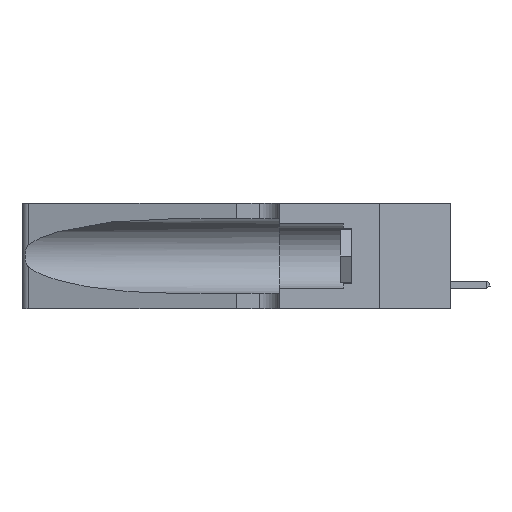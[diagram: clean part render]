
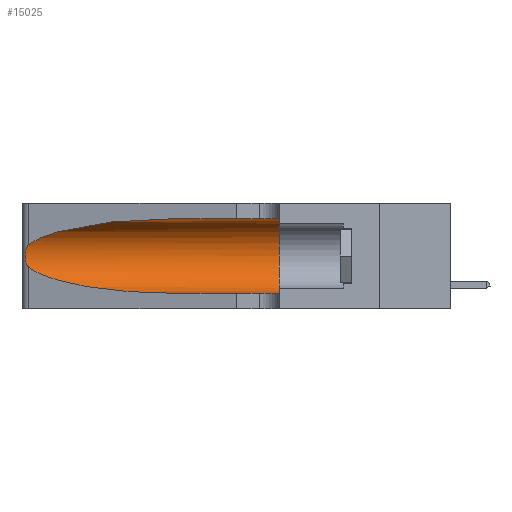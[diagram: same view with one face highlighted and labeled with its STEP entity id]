
A CAD part, left-side view. The second image highlights one B-rep face of the part: STEP entity #15025.
In plain terms, the highlighted cylindrical face has radius 3.308 mm (diameter 6.617 mm), a partial arc.
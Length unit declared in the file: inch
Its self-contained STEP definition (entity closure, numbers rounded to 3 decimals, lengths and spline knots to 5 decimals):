
#577 = CARTESIAN_POINT ( 'NONE',  ( 0.1305, 1.61858, 0.05475 ) ) ;
#926 = CARTESIAN_POINT ( 'NONE',  ( 0.25487, 1.22718, 0.22369 ) ) ;
#1427 = CARTESIAN_POINT ( 'NONE',  ( 0.2373, 1.15595, 0.08982 ) ) ;
#1828 = CARTESIAN_POINT ( 'NONE',  ( 0.25789, 1.23486, 0.15765 ) ) ;
#1886 = CARTESIAN_POINT ( 'NONE',  ( 0.1305, 1.61858, 0.31525 ) ) ;
#2007 = CARTESIAN_POINT ( 'NONE',  ( 0.1305, 0.72297, 0.31525 ) ) ;
#2019 = AXIS2_PLACEMENT_3D ( 'NONE', #18023, #8363, #10877 ) ;
#2122 = EDGE_CURVE ( 'NONE', #17724, #21665, #11173, .T. ) ;
#3225 = CARTESIAN_POINT ( 'NONE',  ( 0.1305, 1.61858, 0.185 ) ) ;
#3258 = EDGE_LOOP ( 'NONE', ( #9719, #6679, #14678, #19673, #24991, #16058 ) ) ;
#5474 = LINE ( 'NONE', #577, #17041 ) ;
#5786 = CARTESIAN_POINT ( 'NONE',  ( 0.25854, 1.2359, 0.20912 ) ) ;
#6450 = AXIS2_PLACEMENT_3D ( 'NONE', #3225, #24688, #18754 ) ;
#6679 = ORIENTED_EDGE ( 'NONE', *, *, #7517, .T. ) ;
#6964 = CARTESIAN_POINT ( 'NONE',  ( 0.1305, 0.35, 0.31525 ) ) ;
#7098 = CARTESIAN_POINT ( 'NONE',  ( 0.18966, 0.96281, 0.05475 ) ) ;
#7517 = EDGE_CURVE ( 'NONE', #14878, #10443, #12636, .T. ) ;
#7521 = CARTESIAN_POINT ( 'NONE',  ( 0.26017, 1.23833, 0.17102 ) ) ;
#7682 = CARTESIAN_POINT ( 'NONE',  ( 0.25856, 1.23593, 0.16098 ) ) ;
#7783 = CARTESIAN_POINT ( 'NONE',  ( 0.18966, 0.96281, 0.31525 ) ) ;
#8119 = CARTESIAN_POINT ( 'NONE',  ( 0.1305, 0.72297, 0.31525 ) ) ;
#8363 = DIRECTION ( 'NONE',  ( 0., 1., 0. ) ) ;
#8421 = FACE_OUTER_BOUND ( 'NONE', #3258, .T. ) ;
#9545 = DIRECTION ( 'NONE',  ( 0., -1., 0. ) ) ;
#9719 = ORIENTED_EDGE ( 'NONE', *, *, #24271, .T. ) ;
#9806 = CARTESIAN_POINT ( 'NONE',  ( 0.25487, 1.22718, 0.14631 ) ) ;
#10043 = EDGE_CURVE ( 'NONE', #21665, #16851, #21026, .T. ) ;
#10149 = EDGE_CURVE ( 'NONE', #14196, #16851, #5474, .T. ) ;
#10443 = VERTEX_POINT ( 'NONE', #12138 ) ;
#10877 = DIRECTION ( 'NONE',  ( 0., 0., 1. ) ) ;
#11173 = LINE ( 'NONE', #1886, #15123 ) ;
#11995 = EDGE_CURVE ( 'NONE', #10443, #14196, #16378, .T. ) ;
#12138 = CARTESIAN_POINT ( 'NONE',  ( 0.25487, 1.22718, 0.14631 ) ) ;
#12348 = CYLINDRICAL_SURFACE ( 'NONE', #6450, 0.13025 ) ;
#12636 = B_SPLINE_CURVE_WITH_KNOTS ( 'NONE', 3,
 ( #17522, #23247, #19146, #19464, #5786, #17267, #23062, #23220, #7521, #7682, #1828, #21189, #21274, #9806 ),
 .UNSPECIFIED., .F., .F.,
 ( 4, 2, 2, 2, 2, 2, 4 ),
 ( 0., 0.00027, 0.00053, 0.00107, 0.0016, 0.00187, 0.00214 ),
 .UNSPECIFIED. ) ;
#14196 = VERTEX_POINT ( 'NONE', #19982 ) ;
#14678 = ORIENTED_EDGE ( 'NONE', *, *, #11995, .T. ) ;
#14878 = VERTEX_POINT ( 'NONE', #926 ) ;
#15025 = ADVANCED_FACE ( 'NONE', ( #8421 ), #12348, .F. ) ;
#15097 = DIRECTION ( 'NONE',  ( 0., -1., 0. ) ) ;
#15123 = VECTOR ( 'NONE', #9545, 39.37008 ) ;
#15824 = CARTESIAN_POINT ( 'NONE',  ( 0.2373, 1.15595, 0.28018 ) ) ;
#16058 = ORIENTED_EDGE ( 'NONE', *, *, #2122, .F. ) ;
#16378 =( BOUNDED_CURVE ( )  B_SPLINE_CURVE ( 3, ( #20607, #1427, #7098, #20696 ),
 .UNSPECIFIED., .F., .F. ) 
 B_SPLINE_CURVE_WITH_KNOTS ( ( 4, 4 ),
 ( 3.44316, 4.71239 ),
 .UNSPECIFIED. ) 
 CURVE ( )  GEOMETRIC_REPRESENTATION_ITEM ( )  RATIONAL_B_SPLINE_CURVE ( ( 1., 0.87, 0.87, 1. ) ) 
 REPRESENTATION_ITEM ( '' )  );
#16851 = VERTEX_POINT ( 'NONE', #18843 ) ;
#17041 = VECTOR ( 'NONE', #15097, 39.37008 ) ;
#17267 = CARTESIAN_POINT ( 'NONE',  ( 0.26018, 1.23835, 0.19895 ) ) ;
#17522 = CARTESIAN_POINT ( 'NONE',  ( 0.25487, 1.22718, 0.22369 ) ) ;
#17724 = VERTEX_POINT ( 'NONE', #8119 ) ;
#18023 = CARTESIAN_POINT ( 'NONE',  ( 0.1305, 0.35, 0.185 ) ) ;
#18705 =( BOUNDED_CURVE ( )  B_SPLINE_CURVE ( 3, ( #2007, #7783, #15824, #19469 ),
 .UNSPECIFIED., .F., .F. ) 
 B_SPLINE_CURVE_WITH_KNOTS ( ( 4, 4 ),
 ( 1.5708, 2.84003 ),
 .UNSPECIFIED. ) 
 CURVE ( )  GEOMETRIC_REPRESENTATION_ITEM ( )  RATIONAL_B_SPLINE_CURVE ( ( 1., 0.87, 0.87, 1. ) ) 
 REPRESENTATION_ITEM ( '' )  );
#18754 = DIRECTION ( 'NONE',  ( 0., 0., -1. ) ) ;
#18843 = CARTESIAN_POINT ( 'NONE',  ( 0.1305, 0.35, 0.05475 ) ) ;
#19146 = CARTESIAN_POINT ( 'NONE',  ( 0.25639, 1.23184, 0.21858 ) ) ;
#19464 = CARTESIAN_POINT ( 'NONE',  ( 0.25787, 1.23484, 0.2124 ) ) ;
#19469 = CARTESIAN_POINT ( 'NONE',  ( 0.25487, 1.22718, 0.22369 ) ) ;
#19673 = ORIENTED_EDGE ( 'NONE', *, *, #10149, .T. ) ;
#19982 = CARTESIAN_POINT ( 'NONE',  ( 0.1305, 0.72297, 0.05475 ) ) ;
#20607 = CARTESIAN_POINT ( 'NONE',  ( 0.25487, 1.22718, 0.14631 ) ) ;
#20696 = CARTESIAN_POINT ( 'NONE',  ( 0.1305, 0.72297, 0.05475 ) ) ;
#21026 = CIRCLE ( 'NONE', #2019, 0.13025 ) ;
#21189 = CARTESIAN_POINT ( 'NONE',  ( 0.25639, 1.23186, 0.15144 ) ) ;
#21274 = CARTESIAN_POINT ( 'NONE',  ( 0.25555, 1.22993, 0.14849 ) ) ;
#21665 = VERTEX_POINT ( 'NONE', #6964 ) ;
#23062 = CARTESIAN_POINT ( 'NONE',  ( 0.26075, 1.23896, 0.19203 ) ) ;
#23220 = CARTESIAN_POINT ( 'NONE',  ( 0.26075, 1.23896, 0.178 ) ) ;
#23247 = CARTESIAN_POINT ( 'NONE',  ( 0.25555, 1.22994, 0.2215 ) ) ;
#24271 = EDGE_CURVE ( 'NONE', #17724, #14878, #18705, .T. ) ;
#24688 = DIRECTION ( 'NONE',  ( 0., -1., 0. ) ) ;
#24991 = ORIENTED_EDGE ( 'NONE', *, *, #10043, .F. ) ;
